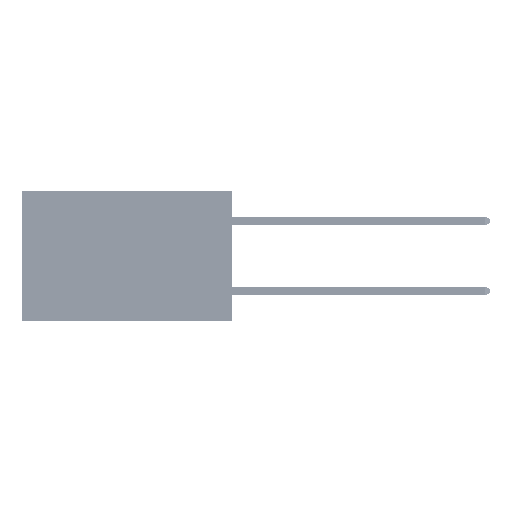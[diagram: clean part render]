
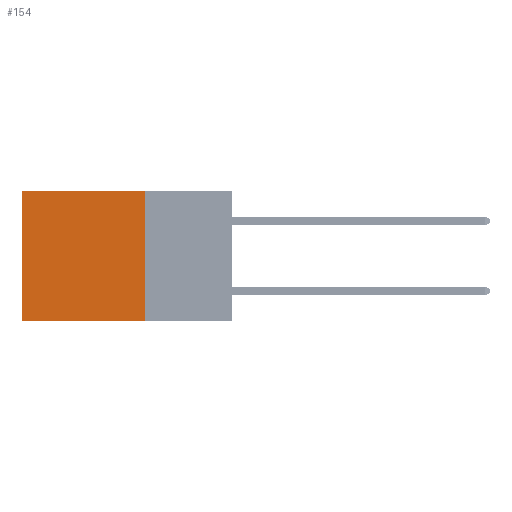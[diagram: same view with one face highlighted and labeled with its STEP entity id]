
A CAD part, left-side view. The second image highlights one B-rep face of the part: STEP entity #154.
In plain terms, the highlighted planar face has unit normal (-1, 0, 0).
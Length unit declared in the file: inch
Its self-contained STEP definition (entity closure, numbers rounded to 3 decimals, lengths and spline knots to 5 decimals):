
#154 = ADVANCED_FACE ( 'NONE', ( #9033 ), #33783, .F. ) ;
#1557 = CARTESIAN_POINT ( 'NONE',  ( 0.2875, 0.25, -0.37 ) ) ;
#1865 = VECTOR ( 'NONE', #25683, 39.37008 ) ;
#4271 = CARTESIAN_POINT ( 'NONE',  ( 0.2875, 0.25, 0. ) ) ;
#4544 = CARTESIAN_POINT ( 'NONE',  ( 0.2875, 0.6, 0. ) ) ;
#5977 = CARTESIAN_POINT ( 'NONE',  ( 0.2875, 0.6, -0.37 ) ) ;
#7425 = CARTESIAN_POINT ( 'NONE',  ( 0.2875, 0.25, 0. ) ) ;
#9033 = FACE_OUTER_BOUND ( 'NONE', #28355, .T. ) ;
#10039 = CARTESIAN_POINT ( 'NONE',  ( 0.2875, 0.25, 0. ) ) ;
#10771 = EDGE_CURVE ( 'NONE', #17244, #51159, #33455, .T. ) ;
#11503 = DIRECTION ( 'NONE',  ( 0., 0., -1. ) ) ;
#12205 = VECTOR ( 'NONE', #11503, 39.37008 ) ;
#14139 = CARTESIAN_POINT ( 'NONE',  ( 0.2875, 0.25, -0.37 ) ) ;
#16494 = ORIENTED_EDGE ( 'NONE', *, *, #10771, .F. ) ;
#17244 = VERTEX_POINT ( 'NONE', #10039 ) ;
#25683 = DIRECTION ( 'NONE',  ( 0., 1., 0. ) ) ;
#26102 = VECTOR ( 'NONE', #28337, 39.37008 ) ;
#26538 = AXIS2_PLACEMENT_3D ( 'NONE', #29785, #49512, #37786 ) ;
#27090 = CARTESIAN_POINT ( 'NONE',  ( 0.2875, 0.6, 0. ) ) ;
#28337 = DIRECTION ( 'NONE',  ( 0., 1., 0. ) ) ;
#28355 = EDGE_LOOP ( 'NONE', ( #35207, #43079, #16494, #49832 ) ) ;
#29785 = CARTESIAN_POINT ( 'NONE',  ( 0.2875, 0.25, 0. ) ) ;
#31376 = VERTEX_POINT ( 'NONE', #27090 ) ;
#32513 = LINE ( 'NONE', #4544, #41817 ) ;
#32637 = LINE ( 'NONE', #1557, #1865 ) ;
#33455 = LINE ( 'NONE', #7425, #12205 ) ;
#33783 = PLANE ( 'NONE',  #26538 ) ;
#34121 = EDGE_CURVE ( 'NONE', #17244, #31376, #45948, .T. ) ;
#35207 = ORIENTED_EDGE ( 'NONE', *, *, #51578, .T. ) ;
#36623 = DIRECTION ( 'NONE',  ( 0., 0., -1. ) ) ;
#37786 = DIRECTION ( 'NONE',  ( 0., 0., -1. ) ) ;
#41817 = VECTOR ( 'NONE', #36623, 39.37008 ) ;
#43079 = ORIENTED_EDGE ( 'NONE', *, *, #43433, .F. ) ;
#43433 = EDGE_CURVE ( 'NONE', #51159, #43467, #32637, .T. ) ;
#43467 = VERTEX_POINT ( 'NONE', #5977 ) ;
#45948 = LINE ( 'NONE', #4271, #26102 ) ;
#49512 = DIRECTION ( 'NONE',  ( 1., 0., 0. ) ) ;
#49832 = ORIENTED_EDGE ( 'NONE', *, *, #34121, .T. ) ;
#51159 = VERTEX_POINT ( 'NONE', #14139 ) ;
#51578 = EDGE_CURVE ( 'NONE', #31376, #43467, #32513, .T. ) ;
